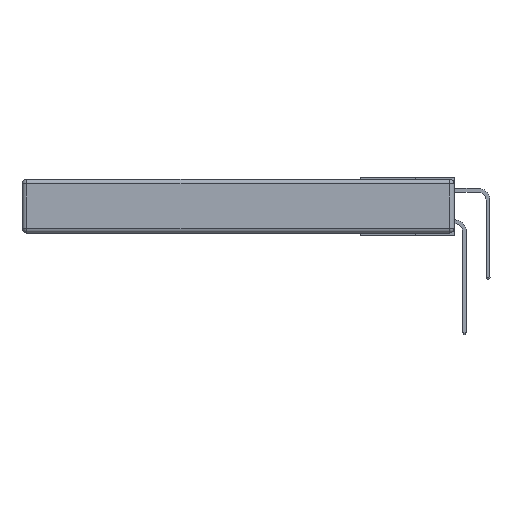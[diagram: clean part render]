
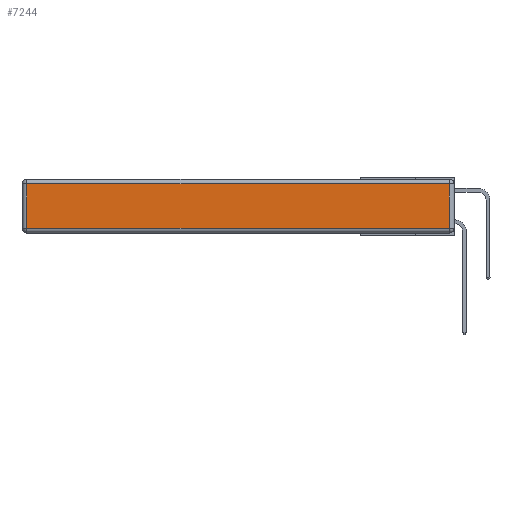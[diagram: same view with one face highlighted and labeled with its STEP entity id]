
A CAD part, left-side view. The second image highlights one B-rep face of the part: STEP entity #7244.
In plain terms, the highlighted planar face has unit normal (-1, 0, 0).
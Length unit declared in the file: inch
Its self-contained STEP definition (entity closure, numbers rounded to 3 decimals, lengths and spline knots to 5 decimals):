
#674 = VERTEX_POINT ( 'NONE', #4663 ) ;
#767 = CARTESIAN_POINT ( 'NONE',  ( 0., 0., -0.343 ) ) ;
#1198 = ORIENTED_EDGE ( 'NONE', *, *, #16263, .T. ) ;
#1545 = VERTEX_POINT ( 'NONE', #26552 ) ;
#4663 = CARTESIAN_POINT ( 'NONE',  ( 0., 2.72, -0.313 ) ) ;
#5576 = EDGE_CURVE ( 'NONE', #674, #31081, #25347, .T. ) ;
#7244 = ADVANCED_FACE ( 'NONE', ( #18796 ), #17420, .T. ) ;
#8357 = VECTOR ( 'NONE', #29181, 39.37008 ) ;
#8954 = LINE ( 'NONE', #24369, #12757 ) ;
#9364 = DIRECTION ( 'NONE',  ( 0., 0., 1. ) ) ;
#10046 = EDGE_CURVE ( 'NONE', #31081, #1545, #17956, .T. ) ;
#11389 = ORIENTED_EDGE ( 'NONE', *, *, #23751, .T. ) ;
#11665 = CARTESIAN_POINT ( 'NONE',  ( 0., 2.72, -0.343 ) ) ;
#12298 = LINE ( 'NONE', #11665, #13844 ) ;
#12757 = VECTOR ( 'NONE', #26787, 39.37008 ) ;
#13310 = ORIENTED_EDGE ( 'NONE', *, *, #10046, .T. ) ;
#13844 = VECTOR ( 'NONE', #30765, 39.37008 ) ;
#15509 = CARTESIAN_POINT ( 'NONE',  ( 0., 0.03, -0.313 ) ) ;
#15725 = CARTESIAN_POINT ( 'NONE',  ( 0., 2.72, -0.03 ) ) ;
#16263 = EDGE_CURVE ( 'NONE', #29415, #674, #12298, .T. ) ;
#17420 = PLANE ( 'NONE',  #17997 ) ;
#17956 = LINE ( 'NONE', #28910, #22875 ) ;
#17997 = AXIS2_PLACEMENT_3D ( 'NONE', #767, #25451, #27697 ) ;
#18796 = FACE_OUTER_BOUND ( 'NONE', #30279, .T. ) ;
#22875 = VECTOR ( 'NONE', #9364, 39.37008 ) ;
#23751 = EDGE_CURVE ( 'NONE', #1545, #29415, #8954, .T. ) ;
#24207 = CARTESIAN_POINT ( 'NONE',  ( 0., 0., -0.313 ) ) ;
#24369 = CARTESIAN_POINT ( 'NONE',  ( 0., 2.75, -0.03 ) ) ;
#24939 = ORIENTED_EDGE ( 'NONE', *, *, #5576, .T. ) ;
#25347 = LINE ( 'NONE', #24207, #8357 ) ;
#25451 = DIRECTION ( 'NONE',  ( -1., 0., 0. ) ) ;
#26552 = CARTESIAN_POINT ( 'NONE',  ( 0., 0.03, -0.03 ) ) ;
#26787 = DIRECTION ( 'NONE',  ( 0., 1., 0. ) ) ;
#27697 = DIRECTION ( 'NONE',  ( 0., 0., 1. ) ) ;
#28910 = CARTESIAN_POINT ( 'NONE',  ( 0., 0.03, -0.343 ) ) ;
#29181 = DIRECTION ( 'NONE',  ( 0., -1., 0. ) ) ;
#29415 = VERTEX_POINT ( 'NONE', #15725 ) ;
#30279 = EDGE_LOOP ( 'NONE', ( #24939, #13310, #11389, #1198 ) ) ;
#30765 = DIRECTION ( 'NONE',  ( 0., 0., -1. ) ) ;
#31081 = VERTEX_POINT ( 'NONE', #15509 ) ;
